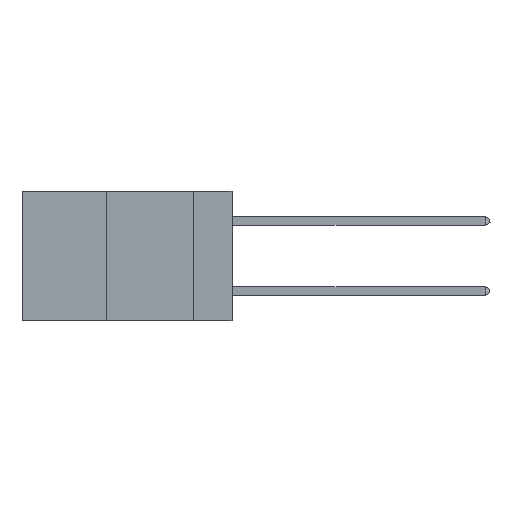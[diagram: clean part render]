
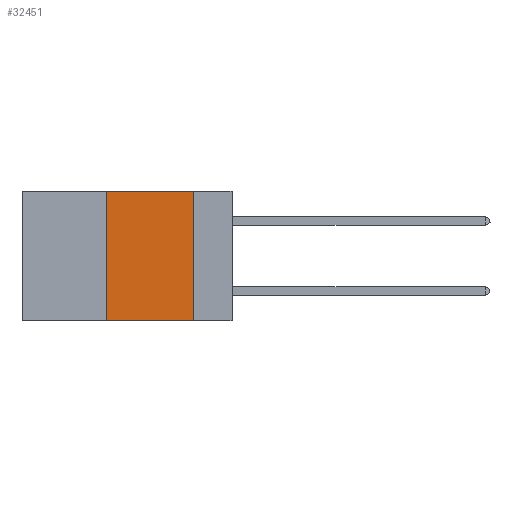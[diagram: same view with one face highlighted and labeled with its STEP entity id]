
A CAD part, left-side view. The second image highlights one B-rep face of the part: STEP entity #32451.
In plain terms, the highlighted planar face has unit normal (-1, 0, 0).
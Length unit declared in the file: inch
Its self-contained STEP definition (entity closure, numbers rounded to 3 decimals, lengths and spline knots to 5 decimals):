
#1289 = CARTESIAN_POINT ( 'NONE',  ( 0., 0.11, 0. ) ) ;
#2410 = PLANE ( 'NONE',  #38855 ) ;
#3407 = VERTEX_POINT ( 'NONE', #15385 ) ;
#3992 = LINE ( 'NONE', #37725, #24306 ) ;
#6365 = DIRECTION ( 'NONE',  ( 1., 0., 0. ) ) ;
#8872 = VERTEX_POINT ( 'NONE', #43195 ) ;
#9772 = CARTESIAN_POINT ( 'NONE',  ( 0., 0.6, -0.37 ) ) ;
#9930 = EDGE_CURVE ( 'NONE', #8872, #47875, #47082, .T. ) ;
#11124 = CARTESIAN_POINT ( 'NONE',  ( 0., 0.36, 0. ) ) ;
#11497 = VECTOR ( 'NONE', #41244, 39.37008 ) ;
#14934 = EDGE_CURVE ( 'NONE', #47875, #3407, #3992, .T. ) ;
#15385 = CARTESIAN_POINT ( 'NONE',  ( 0., 0.11, -0.37 ) ) ;
#16435 = ORIENTED_EDGE ( 'NONE', *, *, #9930, .F. ) ;
#17434 = DIRECTION ( 'NONE',  ( 0., -1., 0. ) ) ;
#18975 = DIRECTION ( 'NONE',  ( 0., 0., -1. ) ) ;
#22338 = ORIENTED_EDGE ( 'NONE', *, *, #34333, .T. ) ;
#23954 = LINE ( 'NONE', #11124, #11497 ) ;
#24306 = VECTOR ( 'NONE', #18975, 39.37008 ) ;
#26290 = CARTESIAN_POINT ( 'NONE',  ( 0., 0.6, 0. ) ) ;
#29122 = CARTESIAN_POINT ( 'NONE',  ( 0., 0.6, 0. ) ) ;
#29330 = LINE ( 'NONE', #9772, #38149 ) ;
#30064 = DIRECTION ( 'NONE',  ( 0., -1., 0. ) ) ;
#30469 = FACE_OUTER_BOUND ( 'NONE', #37826, .T. ) ;
#32451 = ADVANCED_FACE ( 'NONE', ( #30469 ), #2410, .F. ) ;
#32900 = DIRECTION ( 'NONE',  ( 0., 0., -1. ) ) ;
#34117 = ORIENTED_EDGE ( 'NONE', *, *, #14934, .F. ) ;
#34333 = EDGE_CURVE ( 'NONE', #43483, #3407, #29330, .T. ) ;
#35837 = EDGE_CURVE ( 'NONE', #43483, #8872, #23954, .T. ) ;
#37725 = CARTESIAN_POINT ( 'NONE',  ( 0., 0.11, 0. ) ) ;
#37826 = EDGE_LOOP ( 'NONE', ( #34117, #16435, #41126, #22338 ) ) ;
#38149 = VECTOR ( 'NONE', #17434, 39.37008 ) ;
#38855 = AXIS2_PLACEMENT_3D ( 'NONE', #29122, #6365, #32900 ) ;
#41126 = ORIENTED_EDGE ( 'NONE', *, *, #35837, .F. ) ;
#41244 = DIRECTION ( 'NONE',  ( 0., 0., 1. ) ) ;
#43195 = CARTESIAN_POINT ( 'NONE',  ( 0., 0.36, 0. ) ) ;
#43483 = VERTEX_POINT ( 'NONE', #46650 ) ;
#46650 = CARTESIAN_POINT ( 'NONE',  ( 0., 0.36, -0.37 ) ) ;
#47082 = LINE ( 'NONE', #26290, #48256 ) ;
#47875 = VERTEX_POINT ( 'NONE', #1289 ) ;
#48256 = VECTOR ( 'NONE', #30064, 39.37008 ) ;
